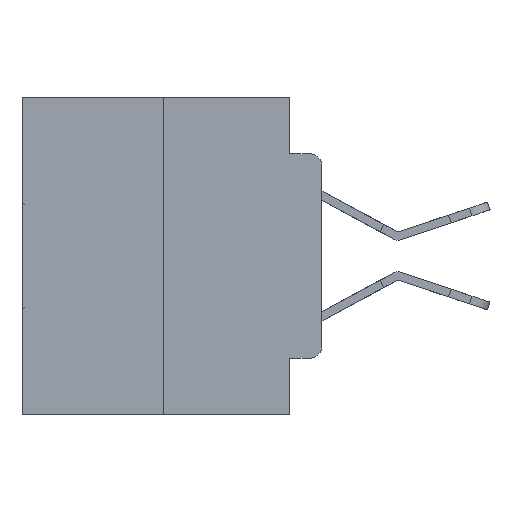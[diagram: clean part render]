
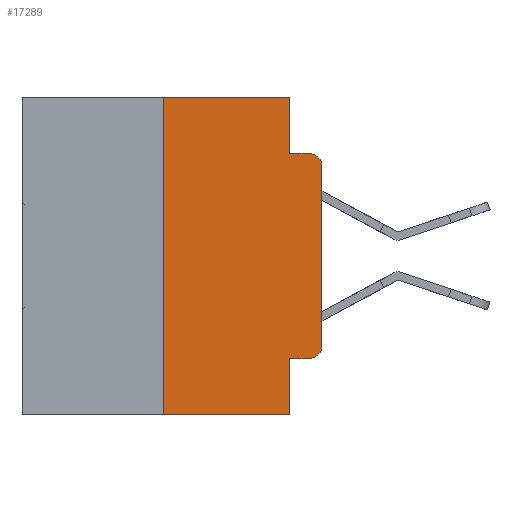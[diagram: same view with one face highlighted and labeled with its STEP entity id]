
A CAD part, left-side view. The second image highlights one B-rep face of the part: STEP entity #17289.
In plain terms, the highlighted planar face has unit normal (-1, 0, 0).
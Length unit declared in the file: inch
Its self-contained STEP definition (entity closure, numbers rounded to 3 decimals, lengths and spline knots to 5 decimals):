
#11 = ORIENTED_EDGE ( 'NONE', *, *, #19798, .F. ) ;
#21 = VERTEX_POINT ( 'NONE', #13672 ) ;
#732 = DIRECTION ( 'NONE',  ( 0., -1., 0. ) ) ;
#1074 = CARTESIAN_POINT ( 'NONE',  ( 0., 0.051, -0.0885 ) ) ;
#1174 = EDGE_CURVE ( 'NONE', #4435, #22694, #18447, .T. ) ;
#1179 = EDGE_CURVE ( 'NONE', #20862, #25528, #1390, .T. ) ;
#1390 = LINE ( 'NONE', #7654, #23812 ) ;
#2400 = VECTOR ( 'NONE', #27870, 39.37008 ) ;
#2663 = CARTESIAN_POINT ( 'NONE',  ( 0., 0.25, -0.5 ) ) ;
#2931 = VERTEX_POINT ( 'NONE', #1074 ) ;
#2949 = ORIENTED_EDGE ( 'NONE', *, *, #17648, .F. ) ;
#3324 = EDGE_CURVE ( 'NONE', #23647, #5488, #25268, .T. ) ;
#3705 = DIRECTION ( 'NONE',  ( -1., 0., 0. ) ) ;
#3890 = DIRECTION ( 'NONE',  ( 0., 0., -1. ) ) ;
#4435 = VERTEX_POINT ( 'NONE', #2663 ) ;
#4661 = EDGE_CURVE ( 'NONE', #6370, #20862, #12215, .T. ) ;
#5212 = CARTESIAN_POINT ( 'NONE',  ( 0., 0.02, -0.4115 ) ) ;
#5479 = CARTESIAN_POINT ( 'NONE',  ( 0., 0.02, -0.3915 ) ) ;
#5488 = VERTEX_POINT ( 'NONE', #22073 ) ;
#5812 = VERTEX_POINT ( 'NONE', #7152 ) ;
#6370 = VERTEX_POINT ( 'NONE', #5212 ) ;
#6978 = VECTOR ( 'NONE', #15786, 39.37008 ) ;
#7035 = CARTESIAN_POINT ( 'NONE',  ( 0., 0.25, 0. ) ) ;
#7152 = CARTESIAN_POINT ( 'NONE',  ( 0., 0.051, -0.4115 ) ) ;
#7343 = DIRECTION ( 'NONE',  ( 0., 0., -1. ) ) ;
#7532 = DIRECTION ( 'NONE',  ( 1., 0., 0. ) ) ;
#7654 = CARTESIAN_POINT ( 'NONE',  ( 0., 0., 0. ) ) ;
#7669 = ORIENTED_EDGE ( 'NONE', *, *, #1174, .T. ) ;
#8607 = CARTESIAN_POINT ( 'NONE',  ( 0., 0., -0.3915 ) ) ;
#8829 = CARTESIAN_POINT ( 'NONE',  ( 0., 0.051, 0. ) ) ;
#9351 = CARTESIAN_POINT ( 'NONE',  ( 0., 0.25, 0. ) ) ;
#9371 = DIRECTION ( 'NONE',  ( 0., 0., 1. ) ) ;
#9399 = CARTESIAN_POINT ( 'NONE',  ( 0., 0.473, 0. ) ) ;
#9475 = CARTESIAN_POINT ( 'NONE',  ( 0., 0.051, -0.0885 ) ) ;
#10487 = DIRECTION ( 'NONE',  ( 0., 0., 1. ) ) ;
#10922 = ORIENTED_EDGE ( 'NONE', *, *, #13552, .F. ) ;
#11732 = FACE_OUTER_BOUND ( 'NONE', #13237, .T. ) ;
#11915 = DIRECTION ( 'NONE',  ( 0., -1., 0. ) ) ;
#11927 = LINE ( 'NONE', #7035, #17349 ) ;
#12215 = CIRCLE ( 'NONE', #19295, 0.02 ) ;
#12269 = VECTOR ( 'NONE', #11915, 39.37008 ) ;
#12290 = CARTESIAN_POINT ( 'NONE',  ( 0., 0.051, -0.4115 ) ) ;
#12840 = CARTESIAN_POINT ( 'NONE',  ( 0., 0.473, -0.5 ) ) ;
#12895 = LINE ( 'NONE', #17753, #18343 ) ;
#13096 = ORIENTED_EDGE ( 'NONE', *, *, #3324, .F. ) ;
#13135 = LINE ( 'NONE', #8829, #6978 ) ;
#13237 = EDGE_LOOP ( 'NONE', ( #27104, #28490, #27802, #10922, #13096, #11, #7669, #2949, #20695, #21403 ) ) ;
#13552 = EDGE_CURVE ( 'NONE', #5488, #2931, #12895, .T. ) ;
#13672 = CARTESIAN_POINT ( 'NONE',  ( 0., 0.02, -0.0885 ) ) ;
#14674 = DIRECTION ( 'NONE',  ( -1., 0., 0. ) ) ;
#15453 = LINE ( 'NONE', #9475, #2400 ) ;
#15786 = DIRECTION ( 'NONE',  ( 0., 0., -1. ) ) ;
#17019 = LINE ( 'NONE', #12290, #20989 ) ;
#17289 = ADVANCED_FACE ( 'NONE', ( #11732 ), #18979, .F. ) ;
#17349 = VECTOR ( 'NONE', #9371, 39.37008 ) ;
#17562 = CARTESIAN_POINT ( 'NONE',  ( 0., 0.02, -0.1085 ) ) ;
#17648 = EDGE_CURVE ( 'NONE', #5812, #22694, #13135, .T. ) ;
#17753 = CARTESIAN_POINT ( 'NONE',  ( 0., 0.051, 0. ) ) ;
#18343 = VECTOR ( 'NONE', #3890, 39.37008 ) ;
#18447 = LINE ( 'NONE', #12840, #12269 ) ;
#18621 = DIRECTION ( 'NONE',  ( 0., -1., 0. ) ) ;
#18857 = EDGE_CURVE ( 'NONE', #25528, #21, #18873, .T. ) ;
#18873 = CIRCLE ( 'NONE', #25111, 0.02 ) ;
#18979 = PLANE ( 'NONE',  #29417 ) ;
#19220 = EDGE_CURVE ( 'NONE', #5812, #6370, #17019, .T. ) ;
#19295 = AXIS2_PLACEMENT_3D ( 'NONE', #5479, #14674, #7343 ) ;
#19798 = EDGE_CURVE ( 'NONE', #4435, #23647, #11927, .T. ) ;
#19911 = DIRECTION ( 'NONE',  ( 0., 0., -1. ) ) ;
#20695 = ORIENTED_EDGE ( 'NONE', *, *, #19220, .T. ) ;
#20862 = VERTEX_POINT ( 'NONE', #8607 ) ;
#20989 = VECTOR ( 'NONE', #732, 39.37008 ) ;
#21362 = CARTESIAN_POINT ( 'NONE',  ( 0., 0.473, 0. ) ) ;
#21403 = ORIENTED_EDGE ( 'NONE', *, *, #4661, .T. ) ;
#22073 = CARTESIAN_POINT ( 'NONE',  ( 0., 0.051, 0. ) ) ;
#22694 = VERTEX_POINT ( 'NONE', #28459 ) ;
#23647 = VERTEX_POINT ( 'NONE', #9351 ) ;
#23677 = DIRECTION ( 'NONE',  ( 0., 0., -1. ) ) ;
#23812 = VECTOR ( 'NONE', #10487, 39.37008 ) ;
#24537 = VECTOR ( 'NONE', #18621, 39.37008 ) ;
#24932 = EDGE_CURVE ( 'NONE', #2931, #21, #15453, .T. ) ;
#25111 = AXIS2_PLACEMENT_3D ( 'NONE', #17562, #3705, #19911 ) ;
#25268 = LINE ( 'NONE', #9399, #24537 ) ;
#25528 = VERTEX_POINT ( 'NONE', #26178 ) ;
#26178 = CARTESIAN_POINT ( 'NONE',  ( 0., 0., -0.1085 ) ) ;
#27104 = ORIENTED_EDGE ( 'NONE', *, *, #1179, .T. ) ;
#27802 = ORIENTED_EDGE ( 'NONE', *, *, #24932, .F. ) ;
#27870 = DIRECTION ( 'NONE',  ( 0., -1., 0. ) ) ;
#28459 = CARTESIAN_POINT ( 'NONE',  ( 0., 0.051, -0.5 ) ) ;
#28490 = ORIENTED_EDGE ( 'NONE', *, *, #18857, .T. ) ;
#29417 = AXIS2_PLACEMENT_3D ( 'NONE', #21362, #7532, #23677 ) ;
